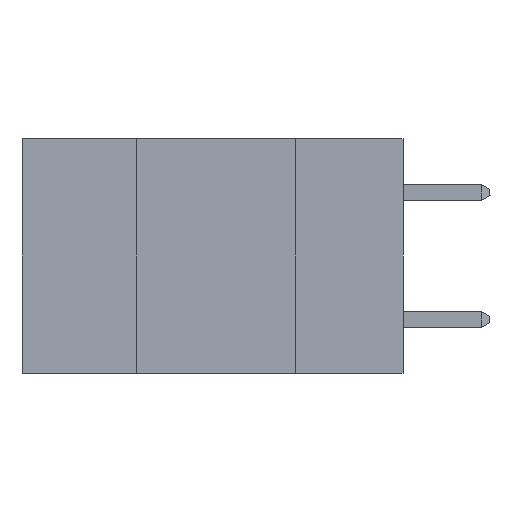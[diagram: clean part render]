
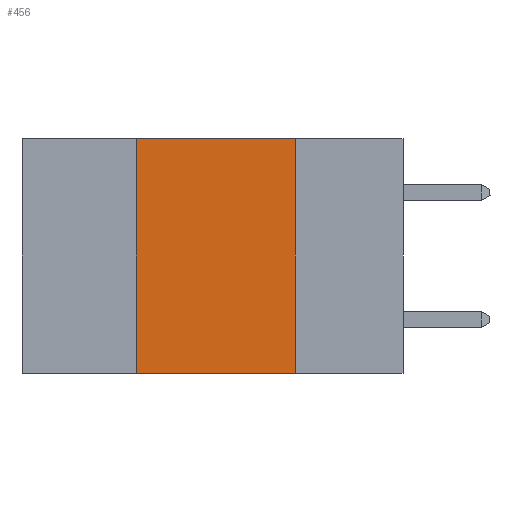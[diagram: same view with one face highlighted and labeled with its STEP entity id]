
A CAD part, left-side view. The second image highlights one B-rep face of the part: STEP entity #456.
In plain terms, the highlighted planar face has unit normal (-1, 0, 0).
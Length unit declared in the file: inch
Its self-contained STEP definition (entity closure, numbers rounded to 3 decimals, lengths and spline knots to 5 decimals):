
#62 = VECTOR ( 'NONE', #16843, 39.37008 ) ;
#456 = ADVANCED_FACE ( 'NONE', ( #34768 ), #25868, .F. ) ;
#474 = CARTESIAN_POINT ( 'NONE',  ( 0., 0.42, 0. ) ) ;
#3205 = ORIENTED_EDGE ( 'NONE', *, *, #22609, .T. ) ;
#5263 = CARTESIAN_POINT ( 'NONE',  ( 0., 0.42, 0. ) ) ;
#5306 = VECTOR ( 'NONE', #23595, 39.37008 ) ;
#5378 = CARTESIAN_POINT ( 'NONE',  ( 0., 0.17, 0. ) ) ;
#5758 = CARTESIAN_POINT ( 'NONE',  ( 0., 0.6, 0. ) ) ;
#6120 = AXIS2_PLACEMENT_3D ( 'NONE', #5758, #14284, #34579 ) ;
#6598 = EDGE_CURVE ( 'NONE', #13615, #17613, #12362, .T. ) ;
#12362 = LINE ( 'NONE', #35502, #36473 ) ;
#12850 = EDGE_CURVE ( 'NONE', #17613, #29746, #28530, .T. ) ;
#13615 = VERTEX_POINT ( 'NONE', #474 ) ;
#14284 = DIRECTION ( 'NONE',  ( 1., 0., 0. ) ) ;
#14346 = ORIENTED_EDGE ( 'NONE', *, *, #6598, .F. ) ;
#16104 = VECTOR ( 'NONE', #30630, 39.37008 ) ;
#16610 = CARTESIAN_POINT ( 'NONE',  ( 0., 0.42, -0.37 ) ) ;
#16843 = DIRECTION ( 'NONE',  ( 0., 0., 1. ) ) ;
#16845 = CARTESIAN_POINT ( 'NONE',  ( 0., 0.17, -0.37 ) ) ;
#17168 = CARTESIAN_POINT ( 'NONE',  ( 0., 0.6, -0.37 ) ) ;
#17613 = VERTEX_POINT ( 'NONE', #5378 ) ;
#19817 = CARTESIAN_POINT ( 'NONE',  ( 0., 0.17, 0. ) ) ;
#22532 = LINE ( 'NONE', #5263, #62 ) ;
#22609 = EDGE_CURVE ( 'NONE', #34559, #29746, #31950, .T. ) ;
#23595 = DIRECTION ( 'NONE',  ( 0., -1., 0. ) ) ;
#24709 = ORIENTED_EDGE ( 'NONE', *, *, #12850, .F. ) ;
#25868 = PLANE ( 'NONE',  #6120 ) ;
#26045 = DIRECTION ( 'NONE',  ( 0., -1., 0. ) ) ;
#26949 = ORIENTED_EDGE ( 'NONE', *, *, #28491, .F. ) ;
#28491 = EDGE_CURVE ( 'NONE', #34559, #13615, #22532, .T. ) ;
#28530 = LINE ( 'NONE', #19817, #16104 ) ;
#29746 = VERTEX_POINT ( 'NONE', #16845 ) ;
#30630 = DIRECTION ( 'NONE',  ( 0., 0., -1. ) ) ;
#31722 = EDGE_LOOP ( 'NONE', ( #24709, #14346, #26949, #3205 ) ) ;
#31950 = LINE ( 'NONE', #17168, #5306 ) ;
#34559 = VERTEX_POINT ( 'NONE', #16610 ) ;
#34579 = DIRECTION ( 'NONE',  ( 0., 0., -1. ) ) ;
#34768 = FACE_OUTER_BOUND ( 'NONE', #31722, .T. ) ;
#35502 = CARTESIAN_POINT ( 'NONE',  ( 0., 0.6, 0. ) ) ;
#36473 = VECTOR ( 'NONE', #26045, 39.37008 ) ;
